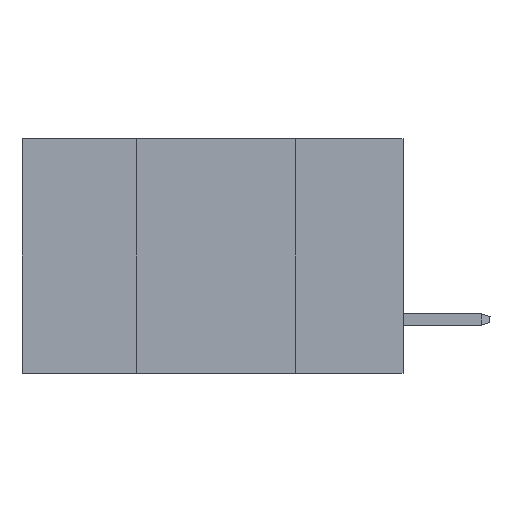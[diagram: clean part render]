
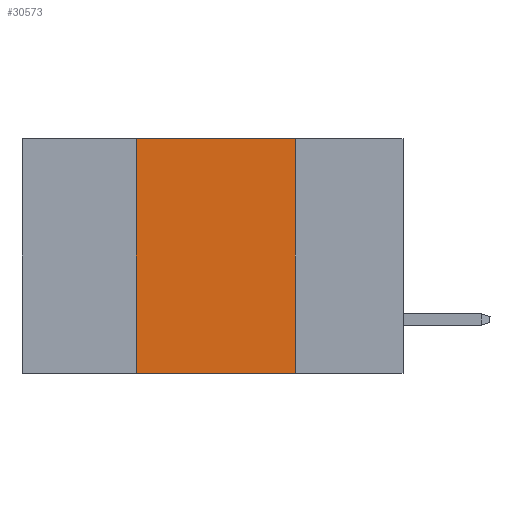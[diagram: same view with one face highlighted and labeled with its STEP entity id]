
A CAD part, left-side view. The second image highlights one B-rep face of the part: STEP entity #30573.
In plain terms, the highlighted planar face has unit normal (-1, 0, 0).
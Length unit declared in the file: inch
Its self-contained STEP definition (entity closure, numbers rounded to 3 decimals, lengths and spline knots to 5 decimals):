
#205 = EDGE_CURVE ( 'NONE', #41943, #17296, #27874, .T. ) ;
#2185 = ORIENTED_EDGE ( 'NONE', *, *, #41160, .F. ) ;
#4127 = DIRECTION ( 'NONE',  ( 0., -1., 0. ) ) ;
#5330 = FACE_OUTER_BOUND ( 'NONE', #8966, .T. ) ;
#5820 = CARTESIAN_POINT ( 'NONE',  ( 0., 0.6, 0. ) ) ;
#6054 = DIRECTION ( 'NONE',  ( 0., 0., -1. ) ) ;
#8846 = ORIENTED_EDGE ( 'NONE', *, *, #30277, .F. ) ;
#8966 = EDGE_LOOP ( 'NONE', ( #28095, #2185, #8846, #31414 ) ) ;
#10175 = DIRECTION ( 'NONE',  ( 0., 0., 1. ) ) ;
#10310 = CARTESIAN_POINT ( 'NONE',  ( 0., 0.17, 0. ) ) ;
#11569 = VERTEX_POINT ( 'NONE', #11578 ) ;
#11578 = CARTESIAN_POINT ( 'NONE',  ( 0., 0.17, 0. ) ) ;
#11980 = VECTOR ( 'NONE', #39487, 39.37008 ) ;
#14372 = VECTOR ( 'NONE', #4127, 39.37008 ) ;
#15443 = LINE ( 'NONE', #38626, #14372 ) ;
#16909 = PLANE ( 'NONE',  #47971 ) ;
#17296 = VERTEX_POINT ( 'NONE', #21584 ) ;
#18615 = LINE ( 'NONE', #10310, #49589 ) ;
#21584 = CARTESIAN_POINT ( 'NONE',  ( 0., 0.17, -0.37 ) ) ;
#21760 = CARTESIAN_POINT ( 'NONE',  ( 0., 0.42, 0. ) ) ;
#21765 = CARTESIAN_POINT ( 'NONE',  ( 0., 0.42, 0. ) ) ;
#25806 = LINE ( 'NONE', #21765, #47196 ) ;
#27874 = LINE ( 'NONE', #35194, #11980 ) ;
#28095 = ORIENTED_EDGE ( 'NONE', *, *, #30623, .F. ) ;
#30277 = EDGE_CURVE ( 'NONE', #41943, #38886, #25806, .T. ) ;
#30573 = ADVANCED_FACE ( 'NONE', ( #5330 ), #16909, .F. ) ;
#30623 = EDGE_CURVE ( 'NONE', #11569, #17296, #18615, .T. ) ;
#31414 = ORIENTED_EDGE ( 'NONE', *, *, #205, .T. ) ;
#32256 = DIRECTION ( 'NONE',  ( 1., 0., 0. ) ) ;
#33221 = DIRECTION ( 'NONE',  ( 0., 0., -1. ) ) ;
#35194 = CARTESIAN_POINT ( 'NONE',  ( 0., 0.6, -0.37 ) ) ;
#38239 = CARTESIAN_POINT ( 'NONE',  ( 0., 0.42, -0.37 ) ) ;
#38626 = CARTESIAN_POINT ( 'NONE',  ( 0., 0.6, 0. ) ) ;
#38886 = VERTEX_POINT ( 'NONE', #21760 ) ;
#39487 = DIRECTION ( 'NONE',  ( 0., -1., 0. ) ) ;
#41160 = EDGE_CURVE ( 'NONE', #38886, #11569, #15443, .T. ) ;
#41943 = VERTEX_POINT ( 'NONE', #38239 ) ;
#47196 = VECTOR ( 'NONE', #10175, 39.37008 ) ;
#47971 = AXIS2_PLACEMENT_3D ( 'NONE', #5820, #32256, #6054 ) ;
#49589 = VECTOR ( 'NONE', #33221, 39.37008 ) ;
